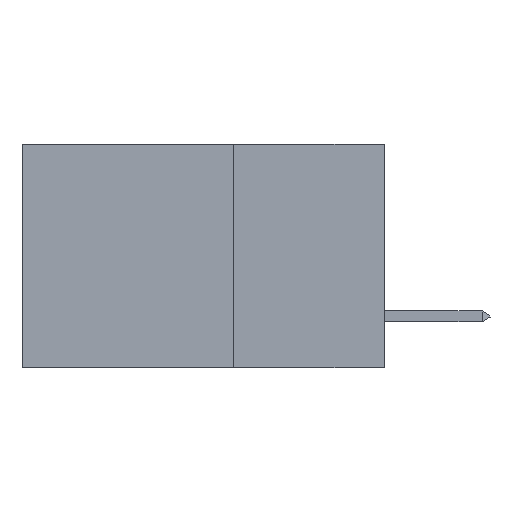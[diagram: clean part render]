
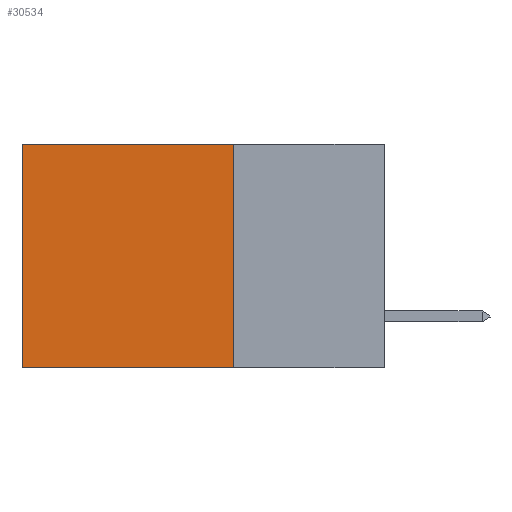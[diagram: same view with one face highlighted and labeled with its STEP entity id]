
A CAD part, left-side view. The second image highlights one B-rep face of the part: STEP entity #30534.
In plain terms, the highlighted planar face has unit normal (-1, 0, 0).
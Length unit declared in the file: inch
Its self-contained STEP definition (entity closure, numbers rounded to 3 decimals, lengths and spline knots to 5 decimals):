
#1 = VECTOR ( 'NONE', #22793, 39.37008 ) ;
#617 = LINE ( 'NONE', #3770, #19758 ) ;
#2107 = CARTESIAN_POINT ( 'NONE',  ( 0.2875, 0.25, 0. ) ) ;
#2545 = VERTEX_POINT ( 'NONE', #30642 ) ;
#3770 = CARTESIAN_POINT ( 'NONE',  ( 0.2875, 0.6, 0. ) ) ;
#4216 = CARTESIAN_POINT ( 'NONE',  ( 0.2875, 0.25, 0. ) ) ;
#5170 = VECTOR ( 'NONE', #30552, 39.37008 ) ;
#5691 = VECTOR ( 'NONE', #20200, 39.37008 ) ;
#5945 = LINE ( 'NONE', #2107, #5170 ) ;
#7610 = LINE ( 'NONE', #8169, #5691 ) ;
#8169 = CARTESIAN_POINT ( 'NONE',  ( 0.2875, 0.25, -0.37 ) ) ;
#8504 = ORIENTED_EDGE ( 'NONE', *, *, #15619, .T. ) ;
#9213 = VERTEX_POINT ( 'NONE', #24527 ) ;
#9576 = ORIENTED_EDGE ( 'NONE', *, *, #25812, .F. ) ;
#11311 = CARTESIAN_POINT ( 'NONE',  ( 0.2875, 0.25, 0. ) ) ;
#13816 = DIRECTION ( 'NONE',  ( 1., 0., 0. ) ) ;
#13830 = VERTEX_POINT ( 'NONE', #11311 ) ;
#13862 = ORIENTED_EDGE ( 'NONE', *, *, #16215, .T. ) ;
#14299 = LINE ( 'NONE', #30154, #1 ) ;
#15619 = EDGE_CURVE ( 'NONE', #13830, #30453, #5945, .T. ) ;
#15798 = CARTESIAN_POINT ( 'NONE',  ( 0.2875, 0.6, 0. ) ) ;
#15893 = FACE_OUTER_BOUND ( 'NONE', #24659, .T. ) ;
#16215 = EDGE_CURVE ( 'NONE', #30453, #2545, #617, .T. ) ;
#17356 = AXIS2_PLACEMENT_3D ( 'NONE', #4216, #13816, #28064 ) ;
#19758 = VECTOR ( 'NONE', #27824, 39.37008 ) ;
#20200 = DIRECTION ( 'NONE',  ( 0., 1., 0. ) ) ;
#20811 = PLANE ( 'NONE',  #17356 ) ;
#22793 = DIRECTION ( 'NONE',  ( 0., 0., -1. ) ) ;
#24527 = CARTESIAN_POINT ( 'NONE',  ( 0.2875, 0.25, -0.37 ) ) ;
#24659 = EDGE_LOOP ( 'NONE', ( #13862, #26630, #9576, #8504 ) ) ;
#25812 = EDGE_CURVE ( 'NONE', #13830, #9213, #14299, .T. ) ;
#26630 = ORIENTED_EDGE ( 'NONE', *, *, #30826, .F. ) ;
#27824 = DIRECTION ( 'NONE',  ( 0., 0., -1. ) ) ;
#28064 = DIRECTION ( 'NONE',  ( 0., 0., -1. ) ) ;
#30154 = CARTESIAN_POINT ( 'NONE',  ( 0.2875, 0.25, 0. ) ) ;
#30453 = VERTEX_POINT ( 'NONE', #15798 ) ;
#30534 = ADVANCED_FACE ( 'NONE', ( #15893 ), #20811, .F. ) ;
#30552 = DIRECTION ( 'NONE',  ( 0., 1., 0. ) ) ;
#30642 = CARTESIAN_POINT ( 'NONE',  ( 0.2875, 0.6, -0.37 ) ) ;
#30826 = EDGE_CURVE ( 'NONE', #9213, #2545, #7610, .T. ) ;
